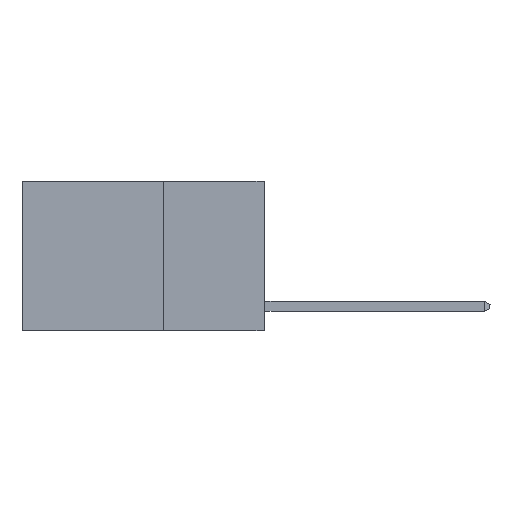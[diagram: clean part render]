
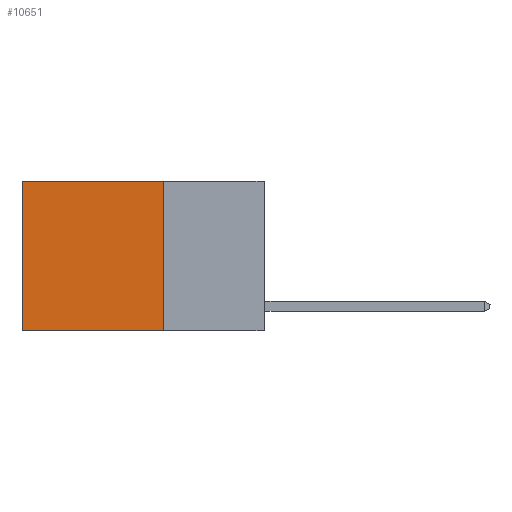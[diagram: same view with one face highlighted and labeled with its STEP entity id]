
A CAD part, left-side view. The second image highlights one B-rep face of the part: STEP entity #10651.
In plain terms, the highlighted planar face has unit normal (-1, 0, 0).
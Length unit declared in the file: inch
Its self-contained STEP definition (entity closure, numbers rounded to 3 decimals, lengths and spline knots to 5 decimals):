
#282 = VECTOR ( 'NONE', #1187, 39.37008 ) ;
#432 = PLANE ( 'NONE',  #8826 ) ;
#1124 = EDGE_CURVE ( 'NONE', #1947, #2323, #10587, .T. ) ;
#1152 = FACE_OUTER_BOUND ( 'NONE', #12259, .T. ) ;
#1187 = DIRECTION ( 'NONE',  ( 0., 1., 0. ) ) ;
#1465 = CARTESIAN_POINT ( 'NONE',  ( 0.2625, 0.25, 0. ) ) ;
#1947 = VERTEX_POINT ( 'NONE', #11335 ) ;
#2323 = VERTEX_POINT ( 'NONE', #3871 ) ;
#3231 = VERTEX_POINT ( 'NONE', #1465 ) ;
#3871 = CARTESIAN_POINT ( 'NONE',  ( 0.2625, 0.6, -0.37 ) ) ;
#4587 = EDGE_CURVE ( 'NONE', #3231, #1947, #7159, .T. ) ;
#4608 = DIRECTION ( 'NONE',  ( 0., 1., 0. ) ) ;
#5721 = EDGE_CURVE ( 'NONE', #3231, #12048, #16204, .T. ) ;
#6840 = CARTESIAN_POINT ( 'NONE',  ( 0.2625, 0.25, 0. ) ) ;
#7159 = LINE ( 'NONE', #16800, #282 ) ;
#7691 = DIRECTION ( 'NONE',  ( 0., 0., -1. ) ) ;
#8134 = VECTOR ( 'NONE', #13207, 39.37008 ) ;
#8826 = AXIS2_PLACEMENT_3D ( 'NONE', #6840, #13451, #10748 ) ;
#8902 = CARTESIAN_POINT ( 'NONE',  ( 0.2625, 0.25, -0.37 ) ) ;
#9389 = ORIENTED_EDGE ( 'NONE', *, *, #1124, .T. ) ;
#9855 = LINE ( 'NONE', #16237, #12676 ) ;
#10587 = LINE ( 'NONE', #15664, #8134 ) ;
#10651 = ADVANCED_FACE ( 'NONE', ( #1152 ), #432, .F. ) ;
#10748 = DIRECTION ( 'NONE',  ( 0., 0., -1. ) ) ;
#11125 = VECTOR ( 'NONE', #7691, 39.37008 ) ;
#11335 = CARTESIAN_POINT ( 'NONE',  ( 0.2625, 0.6, 0. ) ) ;
#11906 = EDGE_CURVE ( 'NONE', #12048, #2323, #9855, .T. ) ;
#12048 = VERTEX_POINT ( 'NONE', #8902 ) ;
#12259 = EDGE_LOOP ( 'NONE', ( #9389, #15145, #15773, #13715 ) ) ;
#12676 = VECTOR ( 'NONE', #4608, 39.37008 ) ;
#13207 = DIRECTION ( 'NONE',  ( 0., 0., -1. ) ) ;
#13451 = DIRECTION ( 'NONE',  ( 1., 0., 0. ) ) ;
#13715 = ORIENTED_EDGE ( 'NONE', *, *, #4587, .T. ) ;
#13898 = CARTESIAN_POINT ( 'NONE',  ( 0.2625, 0.25, 0. ) ) ;
#15145 = ORIENTED_EDGE ( 'NONE', *, *, #11906, .F. ) ;
#15664 = CARTESIAN_POINT ( 'NONE',  ( 0.2625, 0.6, 0. ) ) ;
#15773 = ORIENTED_EDGE ( 'NONE', *, *, #5721, .F. ) ;
#16204 = LINE ( 'NONE', #13898, #11125 ) ;
#16237 = CARTESIAN_POINT ( 'NONE',  ( 0.2625, 0.25, -0.37 ) ) ;
#16800 = CARTESIAN_POINT ( 'NONE',  ( 0.2625, 0.25, 0. ) ) ;
